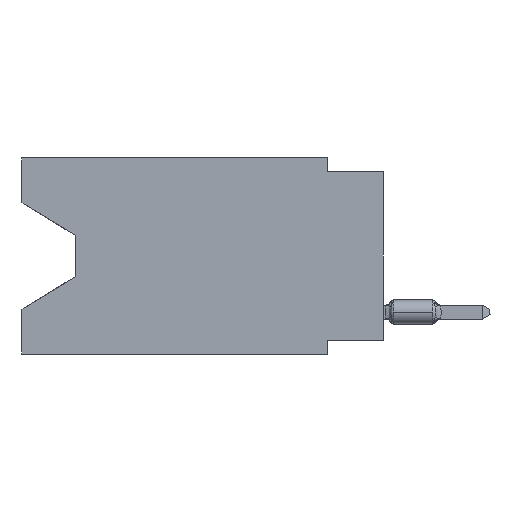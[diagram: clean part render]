
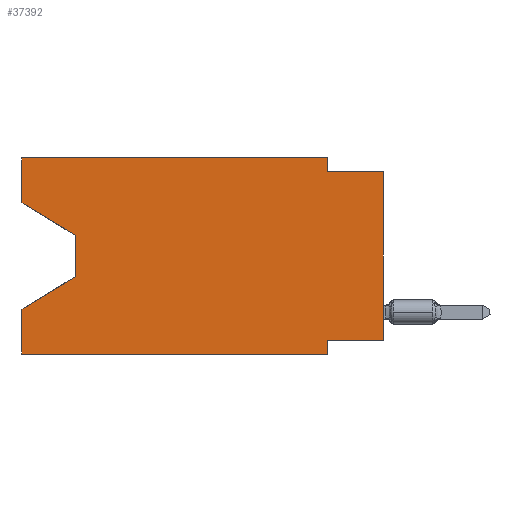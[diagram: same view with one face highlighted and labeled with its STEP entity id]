
A CAD part, left-side view. The second image highlights one B-rep face of the part: STEP entity #37392.
In plain terms, the highlighted planar face has unit normal (-1, 0, 0).
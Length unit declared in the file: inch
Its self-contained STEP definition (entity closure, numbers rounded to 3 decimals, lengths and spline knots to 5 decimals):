
#110 = CARTESIAN_POINT ( 'NONE',  ( 0., 0.645, 0. ) ) ;
#346 = ORIENTED_EDGE ( 'NONE', *, *, #22086, .T. ) ;
#612 = CARTESIAN_POINT ( 'NONE',  ( 0., 0.645, 0. ) ) ;
#1046 = VECTOR ( 'NONE', #30106, 39.37008 ) ;
#1265 = ORIENTED_EDGE ( 'NONE', *, *, #9606, .T. ) ;
#1531 = CARTESIAN_POINT ( 'NONE',  ( 0., 0.1, 0. ) ) ;
#1577 = CARTESIAN_POINT ( 'NONE',  ( 0., 0., 0. ) ) ;
#1959 = EDGE_CURVE ( 'NONE', #10424, #29251, #17353, .T. ) ;
#2073 = VERTEX_POINT ( 'NONE', #15273 ) ;
#2299 = VECTOR ( 'NONE', #23638, 39.37008 ) ;
#2437 = CARTESIAN_POINT ( 'NONE',  ( 0., 0.645, -0.35 ) ) ;
#2589 = ORIENTED_EDGE ( 'NONE', *, *, #15313, .F. ) ;
#2683 = EDGE_CURVE ( 'NONE', #3218, #2073, #22296, .T. ) ;
#2888 = EDGE_CURVE ( 'NONE', #3218, #16288, #40052, .T. ) ;
#3218 = VERTEX_POINT ( 'NONE', #21933 ) ;
#3579 = LINE ( 'NONE', #6696, #36744 ) ;
#3706 = CARTESIAN_POINT ( 'NONE',  ( 0., 0., -0.325 ) ) ;
#3772 = DIRECTION ( 'NONE',  ( 1., 0., 0. ) ) ;
#3796 = DIRECTION ( 'NONE',  ( 0., -1., 0. ) ) ;
#3806 = LINE ( 'NONE', #13615, #16809 ) ;
#4607 = VERTEX_POINT ( 'NONE', #40536 ) ;
#4712 = DIRECTION ( 'NONE',  ( 0., 0., 1. ) ) ;
#6016 = DIRECTION ( 'NONE',  ( 0., 0., -1. ) ) ;
#6452 = ORIENTED_EDGE ( 'NONE', *, *, #27283, .F. ) ;
#6542 = CARTESIAN_POINT ( 'NONE',  ( 0., 0.645, 0. ) ) ;
#6696 = CARTESIAN_POINT ( 'NONE',  ( 0., 0.645, -0.35 ) ) ;
#7708 = DIRECTION ( 'NONE',  ( 0., 0., -1. ) ) ;
#8082 = ORIENTED_EDGE ( 'NONE', *, *, #2888, .T. ) ;
#8967 = CARTESIAN_POINT ( 'NONE',  ( 0., 0.1, -0.35 ) ) ;
#9020 = CARTESIAN_POINT ( 'NONE',  ( 0., 0., -0.025 ) ) ;
#9606 = EDGE_CURVE ( 'NONE', #13555, #4607, #3806, .T. ) ;
#10245 = FACE_OUTER_BOUND ( 'NONE', #22956, .T. ) ;
#10424 = VERTEX_POINT ( 'NONE', #36436 ) ;
#10621 = EDGE_CURVE ( 'NONE', #29251, #13555, #12993, .T. ) ;
#10685 = DIRECTION ( 'NONE',  ( 0., -0.855, -0.519 ) ) ;
#12711 = VECTOR ( 'NONE', #10685, 39.37008 ) ;
#12780 = DIRECTION ( 'NONE',  ( 0., 0., -1. ) ) ;
#12993 = LINE ( 'NONE', #18837, #21433 ) ;
#13136 = EDGE_CURVE ( 'NONE', #24371, #21209, #28401, .T. ) ;
#13251 = DIRECTION ( 'NONE',  ( 0., 0., 1. ) ) ;
#13522 = VERTEX_POINT ( 'NONE', #2437 ) ;
#13555 = VERTEX_POINT ( 'NONE', #28141 ) ;
#13615 = CARTESIAN_POINT ( 'NONE',  ( 0., 0.55, -0.212 ) ) ;
#13636 = CARTESIAN_POINT ( 'NONE',  ( 0., 0.1, -0.35 ) ) ;
#14069 = EDGE_CURVE ( 'NONE', #20205, #24371, #26750, .T. ) ;
#14607 = ORIENTED_EDGE ( 'NONE', *, *, #14069, .F. ) ;
#15273 = CARTESIAN_POINT ( 'NONE',  ( 0., 0.1, -0.325 ) ) ;
#15313 = EDGE_CURVE ( 'NONE', #21209, #16288, #20897, .T. ) ;
#15590 = DIRECTION ( 'NONE',  ( 0., 0., 1. ) ) ;
#15680 = VECTOR ( 'NONE', #17758, 39.37008 ) ;
#16288 = VERTEX_POINT ( 'NONE', #9020 ) ;
#16482 = ORIENTED_EDGE ( 'NONE', *, *, #13136, .F. ) ;
#16809 = VECTOR ( 'NONE', #26353, 39.37008 ) ;
#16823 = CARTESIAN_POINT ( 'NONE',  ( 0., 0.1, -0.025 ) ) ;
#16989 = VECTOR ( 'NONE', #6016, 39.37008 ) ;
#17353 = LINE ( 'NONE', #20488, #12711 ) ;
#17758 = DIRECTION ( 'NONE',  ( 0., -1., 0. ) ) ;
#18173 = EDGE_CURVE ( 'NONE', #13522, #4607, #28920, .T. ) ;
#18565 = CARTESIAN_POINT ( 'NONE',  ( 0., 0.1, 0. ) ) ;
#18837 = CARTESIAN_POINT ( 'NONE',  ( 0., 0.55, -0.138 ) ) ;
#20205 = VERTEX_POINT ( 'NONE', #26493 ) ;
#20488 = CARTESIAN_POINT ( 'NONE',  ( 0., 0.645, -0.08025 ) ) ;
#20897 = LINE ( 'NONE', #33226, #15680 ) ;
#21209 = VERTEX_POINT ( 'NONE', #16823 ) ;
#21433 = VECTOR ( 'NONE', #12780, 39.37008 ) ;
#21933 = CARTESIAN_POINT ( 'NONE',  ( 0., 0., -0.325 ) ) ;
#22086 = EDGE_CURVE ( 'NONE', #13522, #22338, #3579, .T. ) ;
#22296 = LINE ( 'NONE', #3706, #39847 ) ;
#22338 = VERTEX_POINT ( 'NONE', #8967 ) ;
#22956 = EDGE_LOOP ( 'NONE', ( #37479, #32259, #1265, #33394, #346, #24038, #26767, #8082, #2589, #16482, #14607, #6452 ) ) ;
#23638 = DIRECTION ( 'NONE',  ( 0., 0., -1. ) ) ;
#24038 = ORIENTED_EDGE ( 'NONE', *, *, #24770, .F. ) ;
#24371 = VERTEX_POINT ( 'NONE', #1531 ) ;
#24770 = EDGE_CURVE ( 'NONE', #2073, #22338, #29117, .T. ) ;
#26353 = DIRECTION ( 'NONE',  ( 0., 0.855, -0.519 ) ) ;
#26493 = CARTESIAN_POINT ( 'NONE',  ( 0., 0.645, 0. ) ) ;
#26750 = LINE ( 'NONE', #38735, #1046 ) ;
#26767 = ORIENTED_EDGE ( 'NONE', *, *, #2683, .F. ) ;
#27283 = EDGE_CURVE ( 'NONE', #10424, #20205, #35440, .T. ) ;
#28141 = CARTESIAN_POINT ( 'NONE',  ( 0., 0.55, -0.212 ) ) ;
#28169 = DIRECTION ( 'NONE',  ( 0., 1., 0. ) ) ;
#28401 = LINE ( 'NONE', #18565, #16989 ) ;
#28505 = CARTESIAN_POINT ( 'NONE',  ( 0., 0.55, -0.138 ) ) ;
#28662 = AXIS2_PLACEMENT_3D ( 'NONE', #612, #3772, #7708 ) ;
#28920 = LINE ( 'NONE', #6542, #33921 ) ;
#29117 = LINE ( 'NONE', #13636, #2299 ) ;
#29251 = VERTEX_POINT ( 'NONE', #28505 ) ;
#30106 = DIRECTION ( 'NONE',  ( 0., -1., 0. ) ) ;
#31075 = VECTOR ( 'NONE', #15590, 39.37008 ) ;
#32259 = ORIENTED_EDGE ( 'NONE', *, *, #10621, .T. ) ;
#33226 = CARTESIAN_POINT ( 'NONE',  ( 0., 0., -0.025 ) ) ;
#33394 = ORIENTED_EDGE ( 'NONE', *, *, #18173, .F. ) ;
#33921 = VECTOR ( 'NONE', #13251, 39.37008 ) ;
#35440 = LINE ( 'NONE', #110, #31075 ) ;
#35751 = PLANE ( 'NONE',  #28662 ) ;
#36382 = VECTOR ( 'NONE', #4712, 39.37008 ) ;
#36436 = CARTESIAN_POINT ( 'NONE',  ( 0., 0.645, -0.08025 ) ) ;
#36744 = VECTOR ( 'NONE', #3796, 39.37008 ) ;
#37392 = ADVANCED_FACE ( 'NONE', ( #10245 ), #35751, .F. ) ;
#37479 = ORIENTED_EDGE ( 'NONE', *, *, #1959, .T. ) ;
#38735 = CARTESIAN_POINT ( 'NONE',  ( 0., 0.645, 0. ) ) ;
#39847 = VECTOR ( 'NONE', #28169, 39.37008 ) ;
#40052 = LINE ( 'NONE', #1577, #36382 ) ;
#40536 = CARTESIAN_POINT ( 'NONE',  ( 0., 0.645, -0.26975 ) ) ;
